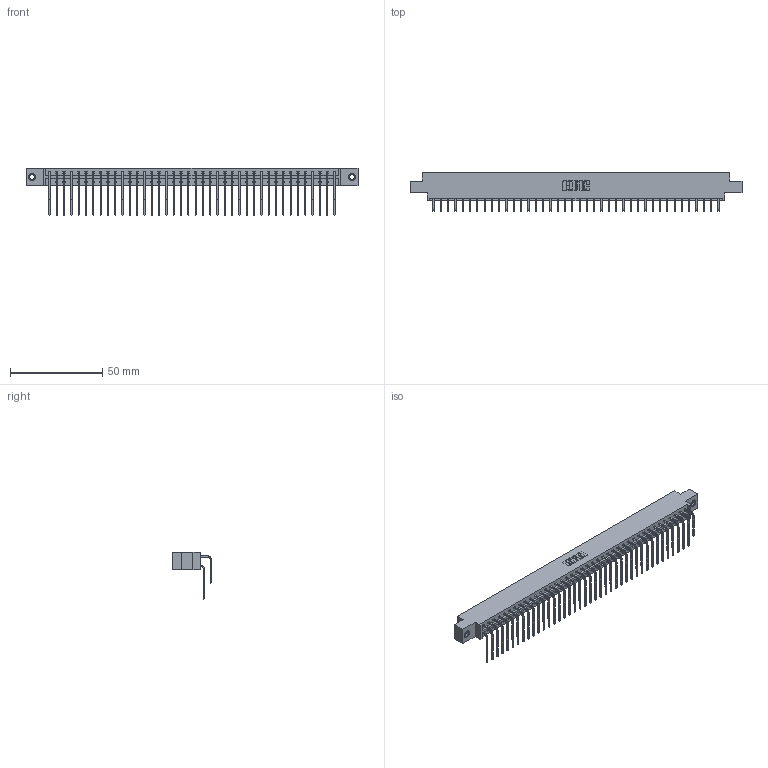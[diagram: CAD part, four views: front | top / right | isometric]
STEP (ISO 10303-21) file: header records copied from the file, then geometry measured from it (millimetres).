
FILE_DESCRIPTION (( 'STEP AP203' ), '1' );
FILE_NAME ('333-080-559-807.STEP', '2018-08-05T02:18:57', ( '' ), ( '' ), 'SwSTEP 2.0', 'SolidWorks 2016', '' );
FILE_SCHEMA (( 'CONFIG_CONTROL_DESIGN' ));
Length unit declared in the file: inch
Products named in the file (5): 345-250-001_345-250-005-103; 333-080-559-807; 333 Part_Offset - .156 Dia - TI; 345-292-001_558 559 Tail - 1; 345-292-001_559 Tail - 2
Assembly tree (83 placements, depth 2):
  333-080-559-807
    333 Part_Offset - .156 Dia - TI
    345-292-001_558 559 Tail - 1  x40
    345-292-001_559 Tail - 2  x40
    345-250-001_345-250-005-103  x2
Bounding box: 180.04 x 20.9 x 25.53 mm (x, y, z)
Volume: 18582.1 mm3; surface area: 24500.8 mm2
Topology: 83 solids, 83 shells, 4498 faces, 13339 edges, 8778 vertices
Faces by surface type: plane 3146, cylinder 1336, cone 12, torus 4
Entity records: 29094 total; most frequent: CARTESIAN_POINT 4860, ORIENTED_EDGE 4738, DIRECTION 4167, EDGE_CURVE 2369, LINE 2181, VECTOR 2181, VERTEX_POINT 1572, AXIS2_PLACEMENT_3D 993
